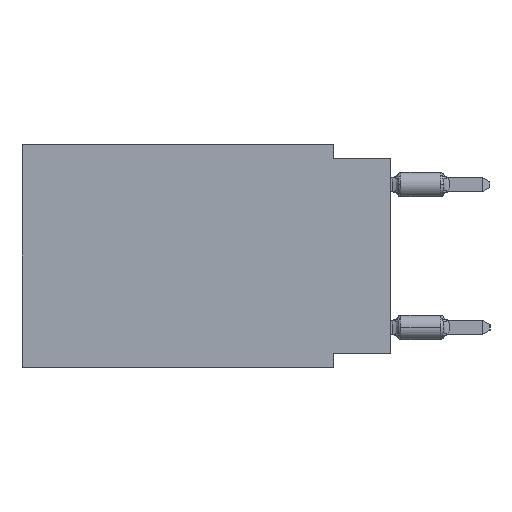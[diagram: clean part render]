
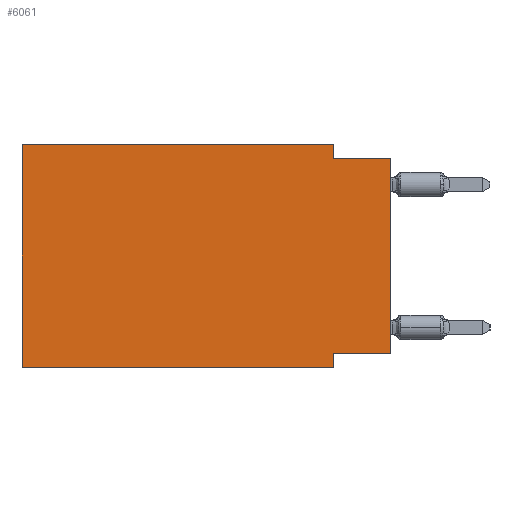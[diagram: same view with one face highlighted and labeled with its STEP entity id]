
A CAD part, left-side view. The second image highlights one B-rep face of the part: STEP entity #6061.
In plain terms, the highlighted planar face has unit normal (-1, 0, 0).
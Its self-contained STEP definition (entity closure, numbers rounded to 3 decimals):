
#786 = DIRECTION ( 'NONE',  ( 0., -1., 0. ) ) ;
#896 = ORIENTED_EDGE ( 'NONE', *, *, #11871, .T. ) ;
#1990 = VECTOR ( 'NONE', #786, 1000. ) ;
#2076 = ORIENTED_EDGE ( 'NONE', *, *, #30241, .F. ) ;
#3867 = EDGE_CURVE ( 'NONE', #54095, #35183, #4830, .T. ) ;
#4830 = LINE ( 'NONE', #34986, #59815 ) ;
#6061 = ADVANCED_FACE ( 'NONE', ( #14700 ), #23566, .F. ) ;
#6828 = CARTESIAN_POINT ( 'NONE',  ( 0., 0., -9.271 ) ) ;
#8336 = LINE ( 'NONE', #38499, #35060 ) ;
#8475 = ORIENTED_EDGE ( 'NONE', *, *, #43522, .F. ) ;
#8711 = AXIS2_PLACEMENT_3D ( 'NONE', #19620, #49161, #9441 ) ;
#9441 = DIRECTION ( 'NONE',  ( 0., 0., -1. ) ) ;
#9618 = CARTESIAN_POINT ( 'NONE',  ( 0., 0., -9.271 ) ) ;
#11871 = EDGE_CURVE ( 'NONE', #54095, #57286, #34558, .T. ) ;
#13517 = CARTESIAN_POINT ( 'NONE',  ( 0., 2.54, -9.271 ) ) ;
#14700 = FACE_OUTER_BOUND ( 'NONE', #46884, .T. ) ;
#15513 = VERTEX_POINT ( 'NONE', #21101 ) ;
#16970 = ORIENTED_EDGE ( 'NONE', *, *, #3867, .F. ) ;
#18181 = DIRECTION ( 'NONE',  ( 0., 0., 1. ) ) ;
#18819 = ORIENTED_EDGE ( 'NONE', *, *, #20855, .F. ) ;
#18979 = LINE ( 'NONE', #37684, #58828 ) ;
#19620 = CARTESIAN_POINT ( 'NONE',  ( 0., 16.383, 0. ) ) ;
#19750 = DIRECTION ( 'NONE',  ( 0., 1., 0. ) ) ;
#20855 = EDGE_CURVE ( 'NONE', #21121, #15513, #62097, .T. ) ;
#21078 = VERTEX_POINT ( 'NONE', #13517 ) ;
#21101 = CARTESIAN_POINT ( 'NONE',  ( 0., 0., -0.635 ) ) ;
#21121 = VERTEX_POINT ( 'NONE', #54854 ) ;
#22065 = DIRECTION ( 'NONE',  ( 0., -1., 0. ) ) ;
#23566 = PLANE ( 'NONE',  #8711 ) ;
#24617 = VECTOR ( 'NONE', #22065, 1000. ) ;
#25079 = DIRECTION ( 'NONE',  ( 0., -1., 0. ) ) ;
#26020 = CARTESIAN_POINT ( 'NONE',  ( 0., 16.383, -9.906 ) ) ;
#29359 = LINE ( 'NONE', #39852, #30622 ) ;
#30241 = EDGE_CURVE ( 'NONE', #40686, #21078, #35464, .T. ) ;
#30622 = VECTOR ( 'NONE', #25079, 1000. ) ;
#31010 = CARTESIAN_POINT ( 'NONE',  ( 0., 16.383, -9.906 ) ) ;
#32221 = CARTESIAN_POINT ( 'NONE',  ( 0., 0., -0.635 ) ) ;
#33080 = DIRECTION ( 'NONE',  ( 0., 0., -1. ) ) ;
#33335 = VECTOR ( 'NONE', #19750, 1000. ) ;
#33756 = EDGE_CURVE ( 'NONE', #21078, #57286, #18979, .T. ) ;
#33944 = ORIENTED_EDGE ( 'NONE', *, *, #51764, .T. ) ;
#34558 = LINE ( 'NONE', #26020, #1990 ) ;
#34959 = CARTESIAN_POINT ( 'NONE',  ( 0., 2.54, 0. ) ) ;
#34986 = CARTESIAN_POINT ( 'NONE',  ( 0., 16.383, 0. ) ) ;
#35060 = VECTOR ( 'NONE', #18181, 1000. ) ;
#35183 = VERTEX_POINT ( 'NONE', #45598 ) ;
#35464 = LINE ( 'NONE', #6828, #33335 ) ;
#35748 = ORIENTED_EDGE ( 'NONE', *, *, #48096, .F. ) ;
#37684 = CARTESIAN_POINT ( 'NONE',  ( 0., 2.54, -9.906 ) ) ;
#38499 = CARTESIAN_POINT ( 'NONE',  ( 0., 0., 0. ) ) ;
#39852 = CARTESIAN_POINT ( 'NONE',  ( 0., 16.383, 0. ) ) ;
#40686 = VERTEX_POINT ( 'NONE', #9618 ) ;
#42796 = DIRECTION ( 'NONE',  ( 0., 0., -1. ) ) ;
#43522 = EDGE_CURVE ( 'NONE', #59288, #21121, #59922, .T. ) ;
#45598 = CARTESIAN_POINT ( 'NONE',  ( 0., 16.383, 0. ) ) ;
#45916 = CARTESIAN_POINT ( 'NONE',  ( 0., 2.54, -9.906 ) ) ;
#46884 = EDGE_LOOP ( 'NONE', ( #33944, #18819, #8475, #35748, #16970, #896, #54990, #2076 ) ) ;
#48096 = EDGE_CURVE ( 'NONE', #35183, #59288, #29359, .T. ) ;
#49161 = DIRECTION ( 'NONE',  ( 1., 0., 0. ) ) ;
#51764 = EDGE_CURVE ( 'NONE', #40686, #15513, #8336, .T. ) ;
#54095 = VERTEX_POINT ( 'NONE', #31010 ) ;
#54854 = CARTESIAN_POINT ( 'NONE',  ( 0., 2.54, -0.635 ) ) ;
#54990 = ORIENTED_EDGE ( 'NONE', *, *, #33756, .F. ) ;
#55043 = DIRECTION ( 'NONE',  ( 0., 0., 1. ) ) ;
#57286 = VERTEX_POINT ( 'NONE', #45916 ) ;
#58664 = VECTOR ( 'NONE', #42796, 1000. ) ;
#58828 = VECTOR ( 'NONE', #33080, 1000. ) ;
#59288 = VERTEX_POINT ( 'NONE', #61138 ) ;
#59815 = VECTOR ( 'NONE', #55043, 1000. ) ;
#59922 = LINE ( 'NONE', #34959, #58664 ) ;
#61138 = CARTESIAN_POINT ( 'NONE',  ( 0., 2.54, 0. ) ) ;
#62097 = LINE ( 'NONE', #32221, #24617 ) ;
